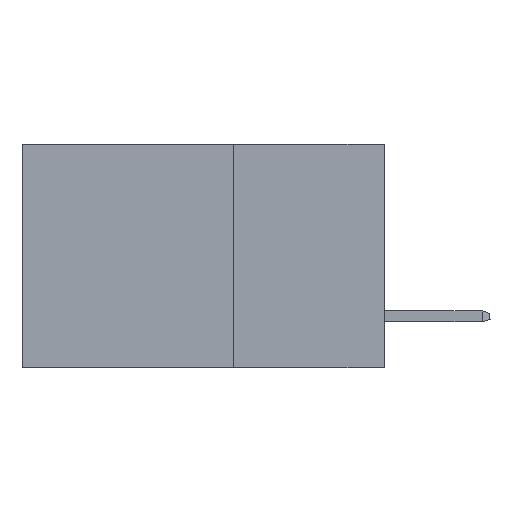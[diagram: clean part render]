
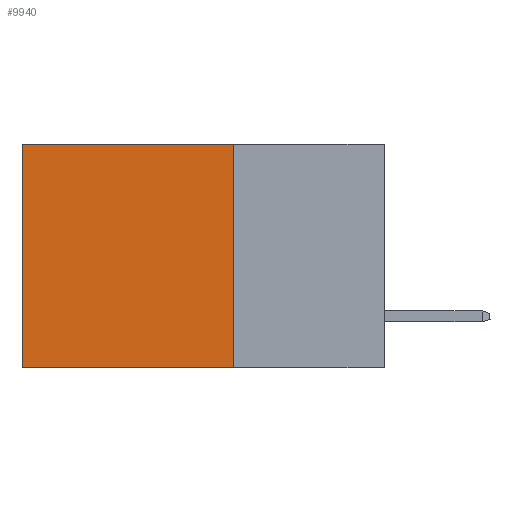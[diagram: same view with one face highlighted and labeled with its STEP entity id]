
A CAD part, left-side view. The second image highlights one B-rep face of the part: STEP entity #9940.
In plain terms, the highlighted planar face has unit normal (-1, 0, 0).
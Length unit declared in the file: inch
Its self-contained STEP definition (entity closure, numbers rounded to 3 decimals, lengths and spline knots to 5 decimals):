
#657 = VERTEX_POINT ( 'NONE', #7631 ) ;
#1077 = EDGE_CURVE ( 'NONE', #4972, #657, #12576, .T. ) ;
#1167 = LINE ( 'NONE', #4940, #3750 ) ;
#1619 = VERTEX_POINT ( 'NONE', #11156 ) ;
#1656 = LINE ( 'NONE', #5459, #11802 ) ;
#2107 = DIRECTION ( 'NONE',  ( 0., 1., 0. ) ) ;
#2192 = DIRECTION ( 'NONE',  ( 0., 0., -1. ) ) ;
#2320 = VERTEX_POINT ( 'NONE', #6096 ) ;
#2985 = EDGE_LOOP ( 'NONE', ( #10739, #6612, #7227, #9059 ) ) ;
#3750 = VECTOR ( 'NONE', #11755, 39.37008 ) ;
#4207 = DIRECTION ( 'NONE',  ( 0., 1., 0. ) ) ;
#4931 = FACE_OUTER_BOUND ( 'NONE', #2985, .T. ) ;
#4940 = CARTESIAN_POINT ( 'NONE',  ( 0.2615, 0.25, -0.37 ) ) ;
#4972 = VERTEX_POINT ( 'NONE', #9286 ) ;
#5162 = DIRECTION ( 'NONE',  ( 0., 0., -1. ) ) ;
#5459 = CARTESIAN_POINT ( 'NONE',  ( 0.2615, 0.25, -0.37 ) ) ;
#5582 = DIRECTION ( 'NONE',  ( 1., 0., 0. ) ) ;
#6096 = CARTESIAN_POINT ( 'NONE',  ( 0.2615, 0.25, -0.37 ) ) ;
#6304 = EDGE_CURVE ( 'NONE', #1619, #2320, #1167, .T. ) ;
#6612 = ORIENTED_EDGE ( 'NONE', *, *, #11635, .F. ) ;
#7227 = ORIENTED_EDGE ( 'NONE', *, *, #6304, .F. ) ;
#7631 = CARTESIAN_POINT ( 'NONE',  ( 0.2615, 0.6, -0.37 ) ) ;
#8529 = CARTESIAN_POINT ( 'NONE',  ( 0.2615, 0.6, -0.37 ) ) ;
#8678 = VECTOR ( 'NONE', #4207, 39.37008 ) ;
#8942 = CARTESIAN_POINT ( 'NONE',  ( 0.2615, 0.25, -0.37 ) ) ;
#9059 = ORIENTED_EDGE ( 'NONE', *, *, #13885, .T. ) ;
#9286 = CARTESIAN_POINT ( 'NONE',  ( 0.2615, 0.6, 0. ) ) ;
#9940 = ADVANCED_FACE ( 'NONE', ( #4931 ), #12032, .F. ) ;
#10569 = LINE ( 'NONE', #11695, #8678 ) ;
#10584 = AXIS2_PLACEMENT_3D ( 'NONE', #8942, #5582, #2192 ) ;
#10739 = ORIENTED_EDGE ( 'NONE', *, *, #1077, .T. ) ;
#11156 = CARTESIAN_POINT ( 'NONE',  ( 0.2615, 0.25, 0. ) ) ;
#11384 = VECTOR ( 'NONE', #5162, 39.37008 ) ;
#11635 = EDGE_CURVE ( 'NONE', #2320, #657, #1656, .T. ) ;
#11695 = CARTESIAN_POINT ( 'NONE',  ( 0.2615, 0.25, 0. ) ) ;
#11755 = DIRECTION ( 'NONE',  ( 0., 0., -1. ) ) ;
#11802 = VECTOR ( 'NONE', #2107, 39.37008 ) ;
#12032 = PLANE ( 'NONE',  #10584 ) ;
#12576 = LINE ( 'NONE', #8529, #11384 ) ;
#13885 = EDGE_CURVE ( 'NONE', #1619, #4972, #10569, .T. ) ;
